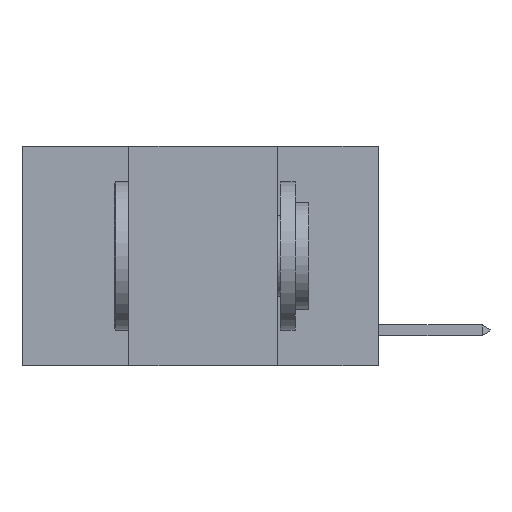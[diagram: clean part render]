
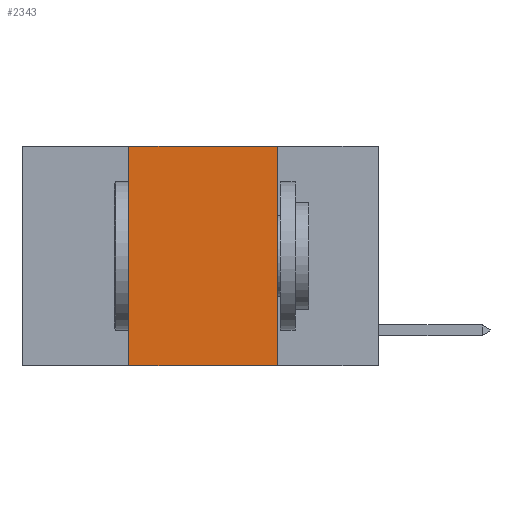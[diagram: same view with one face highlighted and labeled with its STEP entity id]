
A CAD part, left-side view. The second image highlights one B-rep face of the part: STEP entity #2343.
In plain terms, the highlighted planar face has unit normal (-1, 0, 0).
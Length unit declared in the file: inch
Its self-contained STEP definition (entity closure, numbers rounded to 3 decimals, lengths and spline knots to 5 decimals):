
#70 = VERTEX_POINT ( 'NONE', #2219 ) ;
#91 = VERTEX_POINT ( 'NONE', #7023 ) ;
#466 = LINE ( 'NONE', #4240, #4374 ) ;
#859 = DIRECTION ( 'NONE',  ( 0., 0., 1. ) ) ;
#1728 = VERTEX_POINT ( 'NONE', #5071 ) ;
#2219 = CARTESIAN_POINT ( 'NONE',  ( 0., 0.42, -0.37 ) ) ;
#2299 = EDGE_CURVE ( 'NONE', #70, #1728, #6995, .T. ) ;
#2343 = ADVANCED_FACE ( 'NONE', ( #7321 ), #9166, .F. ) ;
#2415 = EDGE_CURVE ( 'NONE', #6371, #91, #466, .T. ) ;
#2520 = VECTOR ( 'NONE', #10624, 39.37008 ) ;
#2855 = CARTESIAN_POINT ( 'NONE',  ( 0., 0.17, 0. ) ) ;
#3651 = CARTESIAN_POINT ( 'NONE',  ( 0., 0.42, 0. ) ) ;
#4240 = CARTESIAN_POINT ( 'NONE',  ( 0., 0.6, 0. ) ) ;
#4296 = VECTOR ( 'NONE', #859, 39.37008 ) ;
#4374 = VECTOR ( 'NONE', #8076, 39.37008 ) ;
#4756 = AXIS2_PLACEMENT_3D ( 'NONE', #10931, #8262, #9103 ) ;
#5071 = CARTESIAN_POINT ( 'NONE',  ( 0., 0.17, -0.37 ) ) ;
#6122 = VECTOR ( 'NONE', #6639, 39.37008 ) ;
#6371 = VERTEX_POINT ( 'NONE', #8032 ) ;
#6639 = DIRECTION ( 'NONE',  ( 0., 0., -1. ) ) ;
#6864 = CARTESIAN_POINT ( 'NONE',  ( 0., 0.6, -0.37 ) ) ;
#6995 = LINE ( 'NONE', #6864, #2520 ) ;
#7023 = CARTESIAN_POINT ( 'NONE',  ( 0., 0.17, 0. ) ) ;
#7321 = FACE_OUTER_BOUND ( 'NONE', #10397, .T. ) ;
#8032 = CARTESIAN_POINT ( 'NONE',  ( 0., 0.42, 0. ) ) ;
#8076 = DIRECTION ( 'NONE',  ( 0., -1., 0. ) ) ;
#8262 = DIRECTION ( 'NONE',  ( 1., 0., 0. ) ) ;
#8394 = ORIENTED_EDGE ( 'NONE', *, *, #2299, .T. ) ;
#9103 = DIRECTION ( 'NONE',  ( 0., 0., -1. ) ) ;
#9166 = PLANE ( 'NONE',  #4756 ) ;
#9372 = ORIENTED_EDGE ( 'NONE', *, *, #2415, .F. ) ;
#9502 = LINE ( 'NONE', #3651, #4296 ) ;
#9644 = ORIENTED_EDGE ( 'NONE', *, *, #11914, .F. ) ;
#10397 = EDGE_LOOP ( 'NONE', ( #9644, #9372, #12068, #8394 ) ) ;
#10552 = EDGE_CURVE ( 'NONE', #70, #6371, #9502, .T. ) ;
#10624 = DIRECTION ( 'NONE',  ( 0., -1., 0. ) ) ;
#10712 = LINE ( 'NONE', #2855, #6122 ) ;
#10931 = CARTESIAN_POINT ( 'NONE',  ( 0., 0.6, 0. ) ) ;
#11914 = EDGE_CURVE ( 'NONE', #91, #1728, #10712, .T. ) ;
#12068 = ORIENTED_EDGE ( 'NONE', *, *, #10552, .F. ) ;
